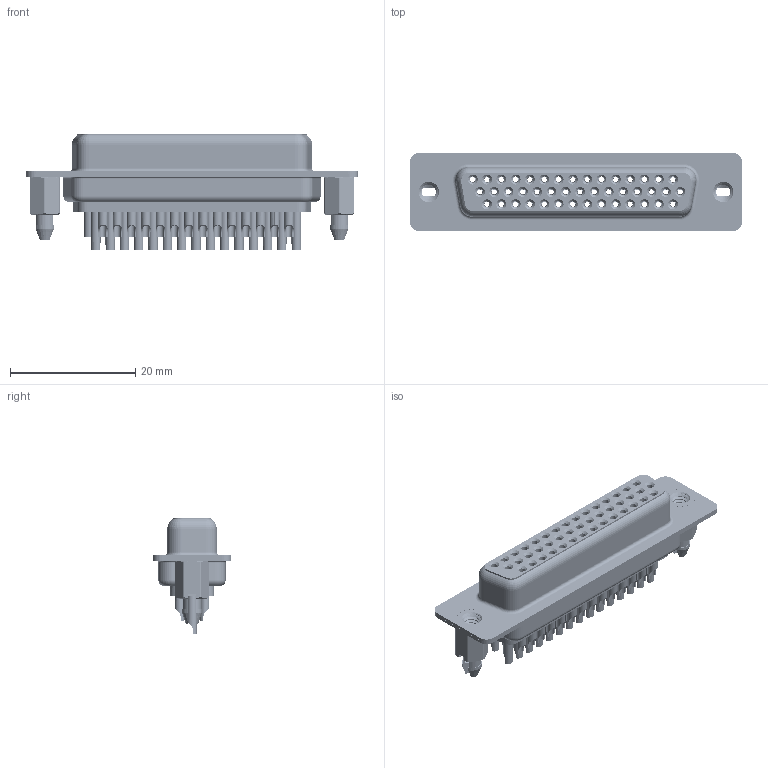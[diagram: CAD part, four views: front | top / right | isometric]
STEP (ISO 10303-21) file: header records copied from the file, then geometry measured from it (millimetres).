
FILE_DESCRIPTION (( 'STEP AP203' ), '1' );
FILE_NAME ('638-044-232-046.STEP', '2020-07-18T22:35:54', ( '' ), ( '' ), 'SwSTEP 2.0', 'SolidWorks 2020', '' );
FILE_SCHEMA (( 'CONFIG_CONTROL_DESIGN' ));
Length unit declared in the file: millimetre
Products named in the file (8): 638-044-232-046; 638 Shell Front_44 Contacts; 638 Shell Rear_44 Contacts; 638 Contact Row 2_32; 638 Contact Row 1_32; 638 4-40 Threaded Boardlock_LP; 638 Contact Row 3_32; 638 Housing_44 Contacts
Assembly tree (49 placements, depth 2):
  638-044-232-046
    638 Housing_44 Contacts
    638 Shell Front_44 Contacts
    638 Shell Rear_44 Contacts
    638 Contact Row 1_32  x15
    638 Contact Row 2_32  x15
    638 Contact Row 3_32  x14
    638 4-40 Threaded Boardlock_LP  x2
Bounding box: 53.04 x 12.6 x 18.6 mm (x, y, z)
Volume: 3457.3 mm3; surface area: 13813.1 mm2
Topology: 49 solids, 49 shells, 4269 faces, 10861 edges, 6831 vertices
Faces by surface type: cylinder 1269, plane 1023, bspline 886, torus 849, cone 242
Entity records: 37149 total; most frequent: CARTESIAN_POINT 9735, DIRECTION 5630, ORIENTED_EDGE 5092, EDGE_CURVE 2546, AXIS2_PLACEMENT_3D 2363, VERTEX_POINT 1617, EDGE_LOOP 1325, CIRCLE 1291
